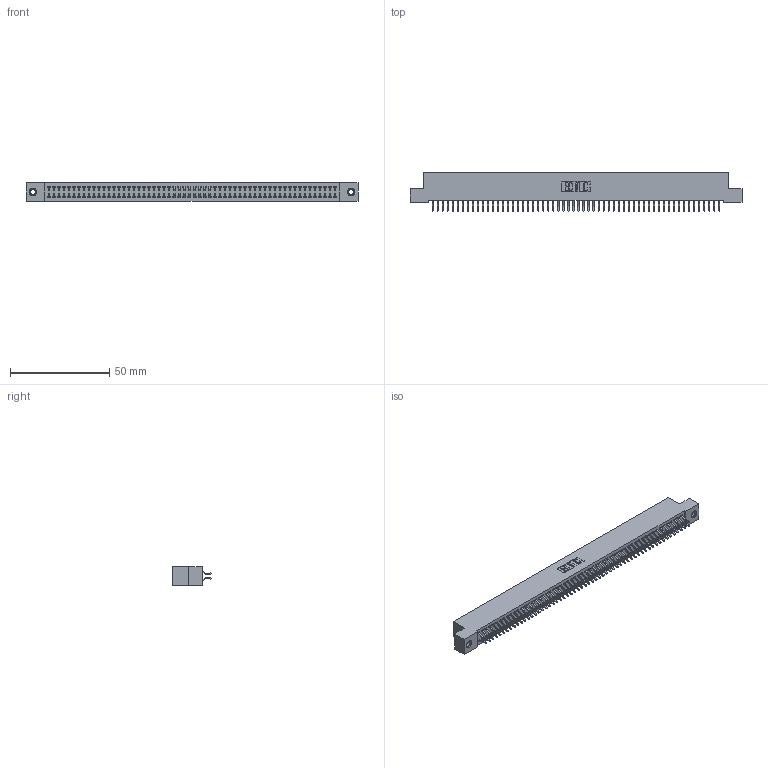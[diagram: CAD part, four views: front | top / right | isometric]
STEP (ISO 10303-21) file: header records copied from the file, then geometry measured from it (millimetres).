
FILE_DESCRIPTION (( 'STEP AP203' ), '1' );
FILE_NAME ('392-116-556-207.STEP', '2019-10-10T01:58:29', ( '' ), ( '' ), 'SwSTEP 2.0', 'SolidWorks 2016', '' );
FILE_SCHEMA (( 'CONFIG_CONTROL_DESIGN' ));
Length unit declared in the file: inch
Products named in the file (4): 342 Part_TI; 345-292-001_556 Tail; 345-250-001_345-250-005-103; 392-116-556-207
Assembly tree (119 placements, depth 2):
  392-116-556-207
    342 Part_TI
    345-292-001_556 Tail  x116
    345-250-001_345-250-005-103  x2
Bounding box: 167.64 x 19.58 x 9.4 mm (x, y, z)
Volume: 15122.5 mm3; surface area: 24923.2 mm2
Topology: 119 solids, 119 shells, 6898 faces, 20503 edges, 13506 vertices
Faces by surface type: plane 4738, cylinder 2144, cone 12, torus 4
Entity records: 36518 total; most frequent: CARTESIAN_POINT 6029, ORIENTED_EDGE 5946, DIRECTION 5143, EDGE_CURVE 2973, VECTOR 2817, LINE 2817, VERTEX_POINT 1976, AXIS2_PLACEMENT_3D 1163
